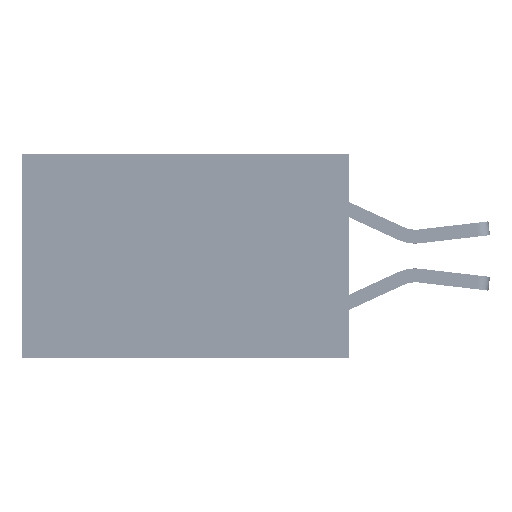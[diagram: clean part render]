
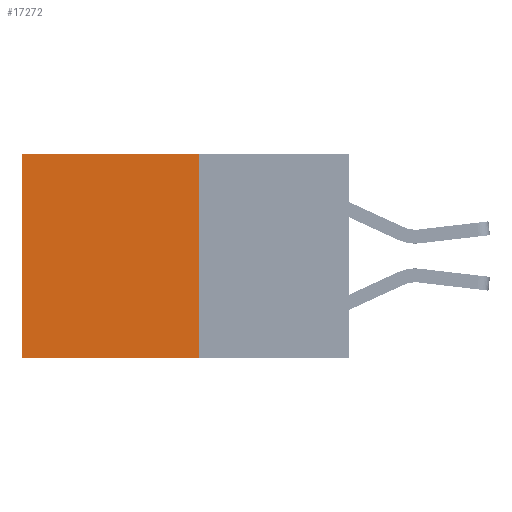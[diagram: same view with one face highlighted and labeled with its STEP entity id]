
A CAD part, left-side view. The second image highlights one B-rep face of the part: STEP entity #17272.
In plain terms, the highlighted planar face has unit normal (-1, 0, 0).
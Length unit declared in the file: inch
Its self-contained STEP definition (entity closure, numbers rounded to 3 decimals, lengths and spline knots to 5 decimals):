
#274 = DIRECTION ( 'NONE',  ( 0., 1., 0. ) ) ;
#831 = VECTOR ( 'NONE', #1406, 39.37008 ) ;
#1252 = VERTEX_POINT ( 'NONE', #16615 ) ;
#1406 = DIRECTION ( 'NONE',  ( 0., 0., -1. ) ) ;
#1635 = LINE ( 'NONE', #11242, #831 ) ;
#2857 = LINE ( 'NONE', #5084, #23476 ) ;
#4116 = EDGE_LOOP ( 'NONE', ( #26152, #11114, #26543, #24855 ) ) ;
#4866 = LINE ( 'NONE', #20201, #10682 ) ;
#5084 = CARTESIAN_POINT ( 'NONE',  ( 0.277, 0.27, -0.37 ) ) ;
#5707 = EDGE_CURVE ( 'NONE', #15653, #25086, #4866, .T. ) ;
#7111 = DIRECTION ( 'NONE',  ( 1., 0., 0. ) ) ;
#10682 = VECTOR ( 'NONE', #20520, 39.37008 ) ;
#11114 = ORIENTED_EDGE ( 'NONE', *, *, #21468, .F. ) ;
#11242 = CARTESIAN_POINT ( 'NONE',  ( 0.277, 0.27, -0.37 ) ) ;
#11797 = VECTOR ( 'NONE', #274, 39.37008 ) ;
#12568 = LINE ( 'NONE', #25171, #11797 ) ;
#14016 = CARTESIAN_POINT ( 'NONE',  ( 0.277, 0.59, 0. ) ) ;
#15547 = FACE_OUTER_BOUND ( 'NONE', #4116, .T. ) ;
#15653 = VERTEX_POINT ( 'NONE', #14016 ) ;
#16033 = AXIS2_PLACEMENT_3D ( 'NONE', #31624, #7111, #24447 ) ;
#16615 = CARTESIAN_POINT ( 'NONE',  ( 0.277, 0.27, -0.37 ) ) ;
#17151 = CARTESIAN_POINT ( 'NONE',  ( 0.277, 0.27, 0. ) ) ;
#17272 = ADVANCED_FACE ( 'NONE', ( #15547 ), #21991, .F. ) ;
#20201 = CARTESIAN_POINT ( 'NONE',  ( 0.277, 0.59, -0.37 ) ) ;
#20520 = DIRECTION ( 'NONE',  ( 0., 0., -1. ) ) ;
#21468 = EDGE_CURVE ( 'NONE', #1252, #25086, #2857, .T. ) ;
#21991 = PLANE ( 'NONE',  #16033 ) ;
#22486 = DIRECTION ( 'NONE',  ( 0., 1., 0. ) ) ;
#22757 = VERTEX_POINT ( 'NONE', #17151 ) ;
#23123 = EDGE_CURVE ( 'NONE', #22757, #1252, #1635, .T. ) ;
#23290 = CARTESIAN_POINT ( 'NONE',  ( 0.277, 0.59, -0.37 ) ) ;
#23476 = VECTOR ( 'NONE', #22486, 39.37008 ) ;
#24447 = DIRECTION ( 'NONE',  ( 0., 0., -1. ) ) ;
#24855 = ORIENTED_EDGE ( 'NONE', *, *, #31996, .T. ) ;
#25086 = VERTEX_POINT ( 'NONE', #23290 ) ;
#25171 = CARTESIAN_POINT ( 'NONE',  ( 0.277, 0.27, 0. ) ) ;
#26152 = ORIENTED_EDGE ( 'NONE', *, *, #5707, .T. ) ;
#26543 = ORIENTED_EDGE ( 'NONE', *, *, #23123, .F. ) ;
#31624 = CARTESIAN_POINT ( 'NONE',  ( 0.277, 0.27, -0.37 ) ) ;
#31996 = EDGE_CURVE ( 'NONE', #22757, #15653, #12568, .T. ) ;
